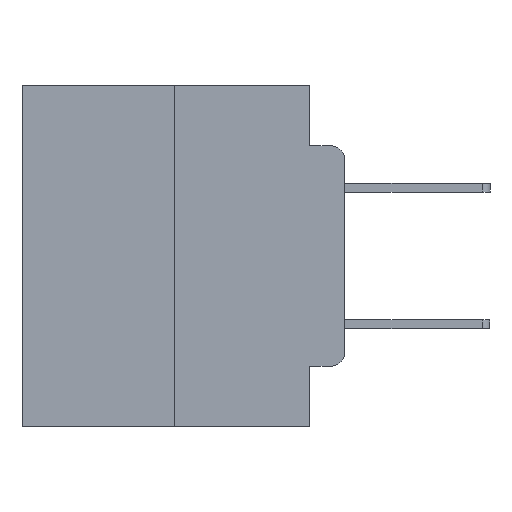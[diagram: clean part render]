
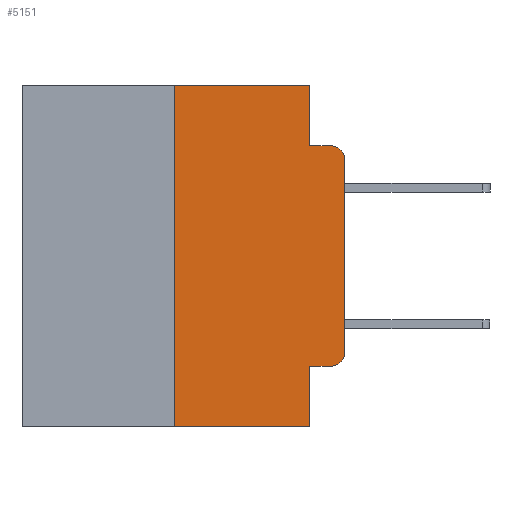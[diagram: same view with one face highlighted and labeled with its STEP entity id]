
A CAD part, left-side view. The second image highlights one B-rep face of the part: STEP entity #5151.
In plain terms, the highlighted planar face has unit normal (-1, 0, 0).
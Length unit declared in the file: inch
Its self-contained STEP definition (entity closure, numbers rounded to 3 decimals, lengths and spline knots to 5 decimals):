
#38 = VERTEX_POINT ( 'NONE', #596 ) ;
#372 = DIRECTION ( 'NONE',  ( 0., -1., 0. ) ) ;
#567 = VERTEX_POINT ( 'NONE', #10615 ) ;
#596 = CARTESIAN_POINT ( 'NONE',  ( 0., 0.02, -0.0885 ) ) ;
#667 = EDGE_CURVE ( 'NONE', #11155, #38, #10042, .T. ) ;
#1399 = ORIENTED_EDGE ( 'NONE', *, *, #18331, .F. ) ;
#1683 = EDGE_LOOP ( 'NONE', ( #18513, #4976, #6568, #1399, #6154, #24462, #16963, #3929, #8211, #5269 ) ) ;
#1958 = EDGE_CURVE ( 'NONE', #567, #14691, #22099, .T. ) ;
#2280 = VERTEX_POINT ( 'NONE', #6008 ) ;
#3174 = CARTESIAN_POINT ( 'NONE',  ( 0., 0.051, -0.0885 ) ) ;
#3385 = DIRECTION ( 'NONE',  ( 0., -1., 0. ) ) ;
#3416 = VECTOR ( 'NONE', #12581, 39.37008 ) ;
#3665 = CIRCLE ( 'NONE', #13820, 0.02 ) ;
#3695 = LINE ( 'NONE', #14658, #13832 ) ;
#3707 = CARTESIAN_POINT ( 'NONE',  ( 0., 0., -0.3915 ) ) ;
#3875 = CARTESIAN_POINT ( 'NONE',  ( 0., 0., 0. ) ) ;
#3929 = ORIENTED_EDGE ( 'NONE', *, *, #24638, .F. ) ;
#4047 = CARTESIAN_POINT ( 'NONE',  ( 0., 0.25, -0.5 ) ) ;
#4052 = EDGE_CURVE ( 'NONE', #4982, #23787, #4849, .T. ) ;
#4116 = CARTESIAN_POINT ( 'NONE',  ( 0., 0.25, 0. ) ) ;
#4190 = FACE_OUTER_BOUND ( 'NONE', #1683, .T. ) ;
#4718 = VECTOR ( 'NONE', #372, 39.37008 ) ;
#4849 = LINE ( 'NONE', #6874, #25595 ) ;
#4976 = ORIENTED_EDGE ( 'NONE', *, *, #667, .T. ) ;
#4982 = VERTEX_POINT ( 'NONE', #4116 ) ;
#5151 = ADVANCED_FACE ( 'NONE', ( #4190 ), #10700, .F. ) ;
#5269 = ORIENTED_EDGE ( 'NONE', *, *, #18820, .T. ) ;
#5275 = VECTOR ( 'NONE', #19027, 39.37008 ) ;
#5906 = LINE ( 'NONE', #14967, #5275 ) ;
#6008 = CARTESIAN_POINT ( 'NONE',  ( 0., 0.051, -0.5 ) ) ;
#6154 = ORIENTED_EDGE ( 'NONE', *, *, #4052, .F. ) ;
#6369 = CARTESIAN_POINT ( 'NONE',  ( 0., 0., -0.1085 ) ) ;
#6568 = ORIENTED_EDGE ( 'NONE', *, *, #12416, .F. ) ;
#6598 = AXIS2_PLACEMENT_3D ( 'NONE', #6978, #6683, #8957 ) ;
#6683 = DIRECTION ( 'NONE',  ( -1., 0., 0. ) ) ;
#6874 = CARTESIAN_POINT ( 'NONE',  ( 0., 0.473, 0. ) ) ;
#6978 = CARTESIAN_POINT ( 'NONE',  ( 0., 0.02, -0.1085 ) ) ;
#8143 = CARTESIAN_POINT ( 'NONE',  ( 0., 0.02, -0.3915 ) ) ;
#8211 = ORIENTED_EDGE ( 'NONE', *, *, #1958, .T. ) ;
#8957 = DIRECTION ( 'NONE',  ( 0., 0., -1. ) ) ;
#9837 = DIRECTION ( 'NONE',  ( 0., 0., 1. ) ) ;
#10037 = LINE ( 'NONE', #20669, #4718 ) ;
#10042 = CIRCLE ( 'NONE', #6598, 0.02 ) ;
#10152 = DIRECTION ( 'NONE',  ( 0., 0., -1. ) ) ;
#10615 = CARTESIAN_POINT ( 'NONE',  ( 0., 0.051, -0.4115 ) ) ;
#10700 = PLANE ( 'NONE',  #14442 ) ;
#11155 = VERTEX_POINT ( 'NONE', #6369 ) ;
#11705 = CARTESIAN_POINT ( 'NONE',  ( 0., 0.051, -0.4115 ) ) ;
#12416 = EDGE_CURVE ( 'NONE', #20256, #38, #10037, .T. ) ;
#12581 = DIRECTION ( 'NONE',  ( 0., 0., -1. ) ) ;
#12738 = DIRECTION ( 'NONE',  ( 0., 0., -1. ) ) ;
#12821 = VERTEX_POINT ( 'NONE', #3707 ) ;
#13230 = LINE ( 'NONE', #15553, #23382 ) ;
#13761 = EDGE_CURVE ( 'NONE', #25827, #4982, #5906, .T. ) ;
#13820 = AXIS2_PLACEMENT_3D ( 'NONE', #8143, #22366, #10152 ) ;
#13832 = VECTOR ( 'NONE', #24685, 39.37008 ) ;
#13902 = VECTOR ( 'NONE', #9837, 39.37008 ) ;
#14442 = AXIS2_PLACEMENT_3D ( 'NONE', #22883, #24834, #12738 ) ;
#14583 = CARTESIAN_POINT ( 'NONE',  ( 0., 0.051, 0. ) ) ;
#14658 = CARTESIAN_POINT ( 'NONE',  ( 0., 0.051, 0. ) ) ;
#14691 = VERTEX_POINT ( 'NONE', #15871 ) ;
#14870 = LINE ( 'NONE', #14583, #3416 ) ;
#14967 = CARTESIAN_POINT ( 'NONE',  ( 0., 0.25, 0. ) ) ;
#15553 = CARTESIAN_POINT ( 'NONE',  ( 0., 0.473, -0.5 ) ) ;
#15871 = CARTESIAN_POINT ( 'NONE',  ( 0., 0.02, -0.4115 ) ) ;
#16709 = VECTOR ( 'NONE', #20515, 39.37008 ) ;
#16963 = ORIENTED_EDGE ( 'NONE', *, *, #24910, .T. ) ;
#16992 = DIRECTION ( 'NONE',  ( 0., -1., 0. ) ) ;
#18331 = EDGE_CURVE ( 'NONE', #23787, #20256, #3695, .T. ) ;
#18513 = ORIENTED_EDGE ( 'NONE', *, *, #24428, .T. ) ;
#18820 = EDGE_CURVE ( 'NONE', #14691, #12821, #3665, .T. ) ;
#19027 = DIRECTION ( 'NONE',  ( 0., 0., 1. ) ) ;
#19950 = CARTESIAN_POINT ( 'NONE',  ( 0., 0.051, 0. ) ) ;
#20256 = VERTEX_POINT ( 'NONE', #3174 ) ;
#20515 = DIRECTION ( 'NONE',  ( 0., -1., 0. ) ) ;
#20669 = CARTESIAN_POINT ( 'NONE',  ( 0., 0.051, -0.0885 ) ) ;
#22099 = LINE ( 'NONE', #11705, #16709 ) ;
#22366 = DIRECTION ( 'NONE',  ( -1., 0., 0. ) ) ;
#22883 = CARTESIAN_POINT ( 'NONE',  ( 0., 0.473, 0. ) ) ;
#23382 = VECTOR ( 'NONE', #3385, 39.37008 ) ;
#23787 = VERTEX_POINT ( 'NONE', #19950 ) ;
#24008 = LINE ( 'NONE', #3875, #13902 ) ;
#24428 = EDGE_CURVE ( 'NONE', #12821, #11155, #24008, .T. ) ;
#24462 = ORIENTED_EDGE ( 'NONE', *, *, #13761, .F. ) ;
#24638 = EDGE_CURVE ( 'NONE', #567, #2280, #14870, .T. ) ;
#24685 = DIRECTION ( 'NONE',  ( 0., 0., -1. ) ) ;
#24834 = DIRECTION ( 'NONE',  ( 1., 0., 0. ) ) ;
#24910 = EDGE_CURVE ( 'NONE', #25827, #2280, #13230, .T. ) ;
#25595 = VECTOR ( 'NONE', #16992, 39.37008 ) ;
#25827 = VERTEX_POINT ( 'NONE', #4047 ) ;
